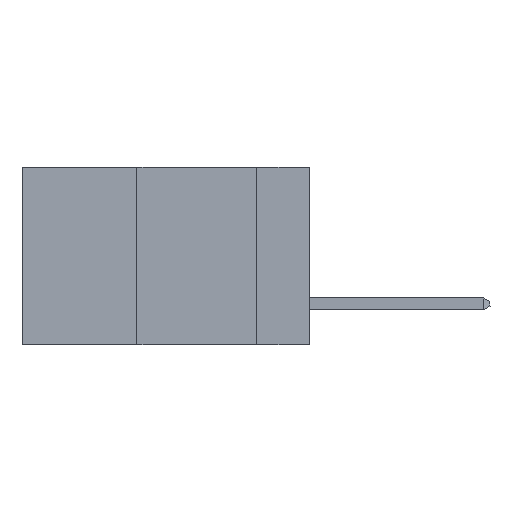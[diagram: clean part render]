
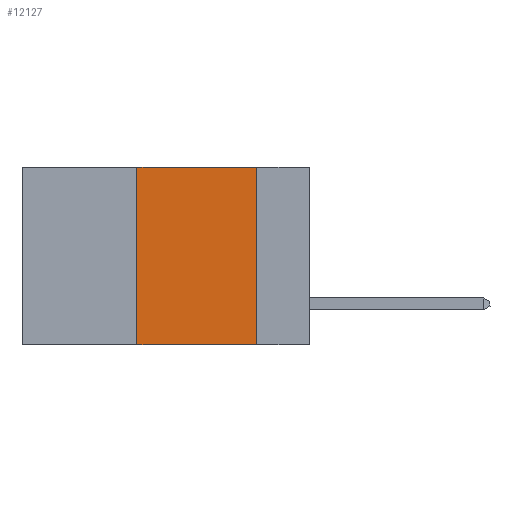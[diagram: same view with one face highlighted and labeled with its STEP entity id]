
A CAD part, left-side view. The second image highlights one B-rep face of the part: STEP entity #12127.
In plain terms, the highlighted planar face has unit normal (-1, 0, 0).
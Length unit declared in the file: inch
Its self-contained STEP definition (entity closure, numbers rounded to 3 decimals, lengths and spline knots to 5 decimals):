
#481 = VERTEX_POINT ( 'NONE', #11432 ) ;
#758 = AXIS2_PLACEMENT_3D ( 'NONE', #4174, #6270, #2241 ) ;
#1193 = CARTESIAN_POINT ( 'NONE',  ( 0., 0.36, 0. ) ) ;
#1686 = ORIENTED_EDGE ( 'NONE', *, *, #10929, .F. ) ;
#1720 = VERTEX_POINT ( 'NONE', #6639 ) ;
#1826 = VERTEX_POINT ( 'NONE', #1193 ) ;
#2184 = DIRECTION ( 'NONE',  ( 0., 0., 1. ) ) ;
#2241 = DIRECTION ( 'NONE',  ( 0., 0., -1. ) ) ;
#2448 = DIRECTION ( 'NONE',  ( 0., 0., -1. ) ) ;
#2707 = VERTEX_POINT ( 'NONE', #10313 ) ;
#3172 = VECTOR ( 'NONE', #11262, 39.37008 ) ;
#4047 = DIRECTION ( 'NONE',  ( 0., -1., 0. ) ) ;
#4174 = CARTESIAN_POINT ( 'NONE',  ( 0., 0.6, 0. ) ) ;
#4326 = LINE ( 'NONE', #10533, #12234 ) ;
#4417 = ORIENTED_EDGE ( 'NONE', *, *, #7110, .T. ) ;
#4888 = CARTESIAN_POINT ( 'NONE',  ( 0., 0.36, 0. ) ) ;
#5031 = VECTOR ( 'NONE', #2184, 39.37008 ) ;
#5174 = FACE_OUTER_BOUND ( 'NONE', #12548, .T. ) ;
#6270 = DIRECTION ( 'NONE',  ( 1., 0., 0. ) ) ;
#6288 = EDGE_CURVE ( 'NONE', #2707, #481, #6521, .T. ) ;
#6321 = CARTESIAN_POINT ( 'NONE',  ( 0., 0.11, 0. ) ) ;
#6521 = LINE ( 'NONE', #6321, #11462 ) ;
#6639 = CARTESIAN_POINT ( 'NONE',  ( 0., 0.36, -0.37 ) ) ;
#7110 = EDGE_CURVE ( 'NONE', #1720, #481, #4326, .T. ) ;
#7903 = ORIENTED_EDGE ( 'NONE', *, *, #6288, .F. ) ;
#9677 = ORIENTED_EDGE ( 'NONE', *, *, #11465, .F. ) ;
#10313 = CARTESIAN_POINT ( 'NONE',  ( 0., 0.11, 0. ) ) ;
#10533 = CARTESIAN_POINT ( 'NONE',  ( 0., 0.6, -0.37 ) ) ;
#10587 = LINE ( 'NONE', #11303, #3172 ) ;
#10929 = EDGE_CURVE ( 'NONE', #1826, #2707, #10587, .T. ) ;
#10958 = PLANE ( 'NONE',  #758 ) ;
#11262 = DIRECTION ( 'NONE',  ( 0., -1., 0. ) ) ;
#11303 = CARTESIAN_POINT ( 'NONE',  ( 0., 0.6, 0. ) ) ;
#11432 = CARTESIAN_POINT ( 'NONE',  ( 0., 0.11, -0.37 ) ) ;
#11462 = VECTOR ( 'NONE', #2448, 39.37008 ) ;
#11465 = EDGE_CURVE ( 'NONE', #1720, #1826, #12169, .T. ) ;
#12127 = ADVANCED_FACE ( 'NONE', ( #5174 ), #10958, .F. ) ;
#12169 = LINE ( 'NONE', #4888, #5031 ) ;
#12234 = VECTOR ( 'NONE', #4047, 39.37008 ) ;
#12548 = EDGE_LOOP ( 'NONE', ( #7903, #1686, #9677, #4417 ) ) ;
